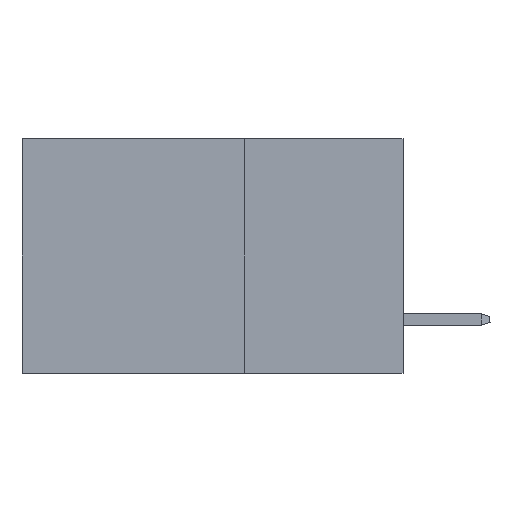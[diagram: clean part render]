
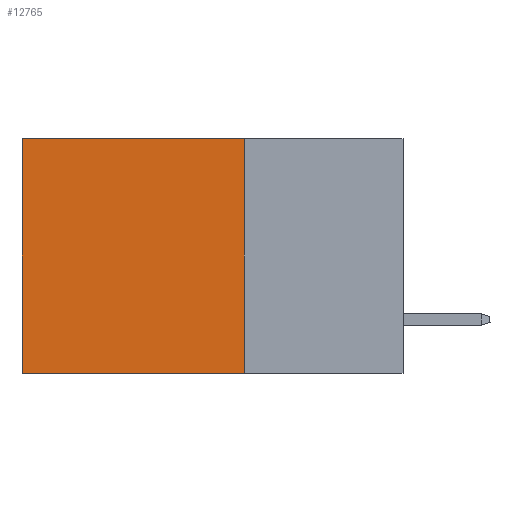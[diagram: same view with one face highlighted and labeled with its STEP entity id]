
A CAD part, left-side view. The second image highlights one B-rep face of the part: STEP entity #12765.
In plain terms, the highlighted planar face has unit normal (-1, 0, 0).
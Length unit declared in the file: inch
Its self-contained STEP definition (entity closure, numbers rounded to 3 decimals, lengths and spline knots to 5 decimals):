
#497 = VERTEX_POINT ( 'NONE', #9409 ) ;
#673 = DIRECTION ( 'NONE',  ( 1., 0., 0. ) ) ;
#829 = ORIENTED_EDGE ( 'NONE', *, *, #5752, .T. ) ;
#1745 = DIRECTION ( 'NONE',  ( 0., 0., -1. ) ) ;
#2105 = VERTEX_POINT ( 'NONE', #18068 ) ;
#2307 = CARTESIAN_POINT ( 'NONE',  ( 0.2875, 0.25, 0. ) ) ;
#3351 = EDGE_CURVE ( 'NONE', #2105, #7802, #7999, .T. ) ;
#3520 = ORIENTED_EDGE ( 'NONE', *, *, #3351, .T. ) ;
#3522 = PLANE ( 'NONE',  #9648 ) ;
#3585 = DIRECTION ( 'NONE',  ( 0., 0., -1. ) ) ;
#4759 = VERTEX_POINT ( 'NONE', #15903 ) ;
#4969 = CARTESIAN_POINT ( 'NONE',  ( 0.2875, 0.25, -0.37 ) ) ;
#5415 = EDGE_CURVE ( 'NONE', #4759, #7802, #9387, .T. ) ;
#5637 = LINE ( 'NONE', #2307, #17193 ) ;
#5752 = EDGE_CURVE ( 'NONE', #497, #2105, #11920, .T. ) ;
#7222 = VECTOR ( 'NONE', #13572, 39.37008 ) ;
#7802 = VERTEX_POINT ( 'NONE', #14185 ) ;
#7999 = LINE ( 'NONE', #9565, #10766 ) ;
#8291 = DIRECTION ( 'NONE',  ( 0., 0., -1. ) ) ;
#8357 = ORIENTED_EDGE ( 'NONE', *, *, #5415, .F. ) ;
#9387 = LINE ( 'NONE', #4969, #16496 ) ;
#9409 = CARTESIAN_POINT ( 'NONE',  ( 0.2875, 0.25, 0. ) ) ;
#9565 = CARTESIAN_POINT ( 'NONE',  ( 0.2875, 0.6, 0. ) ) ;
#9648 = AXIS2_PLACEMENT_3D ( 'NONE', #14081, #673, #1745 ) ;
#10766 = VECTOR ( 'NONE', #3585, 39.37008 ) ;
#11920 = LINE ( 'NONE', #13662, #7222 ) ;
#12330 = FACE_OUTER_BOUND ( 'NONE', #17126, .T. ) ;
#12765 = ADVANCED_FACE ( 'NONE', ( #12330 ), #3522, .F. ) ;
#13572 = DIRECTION ( 'NONE',  ( 0., 1., 0. ) ) ;
#13662 = CARTESIAN_POINT ( 'NONE',  ( 0.2875, 0.25, 0. ) ) ;
#13976 = DIRECTION ( 'NONE',  ( 0., 1., 0. ) ) ;
#14081 = CARTESIAN_POINT ( 'NONE',  ( 0.2875, 0.25, 0. ) ) ;
#14185 = CARTESIAN_POINT ( 'NONE',  ( 0.2875, 0.6, -0.37 ) ) ;
#14385 = ORIENTED_EDGE ( 'NONE', *, *, #15205, .F. ) ;
#15205 = EDGE_CURVE ( 'NONE', #497, #4759, #5637, .T. ) ;
#15903 = CARTESIAN_POINT ( 'NONE',  ( 0.2875, 0.25, -0.37 ) ) ;
#16496 = VECTOR ( 'NONE', #13976, 39.37008 ) ;
#17126 = EDGE_LOOP ( 'NONE', ( #3520, #8357, #14385, #829 ) ) ;
#17193 = VECTOR ( 'NONE', #8291, 39.37008 ) ;
#18068 = CARTESIAN_POINT ( 'NONE',  ( 0.2875, 0.6, 0. ) ) ;
